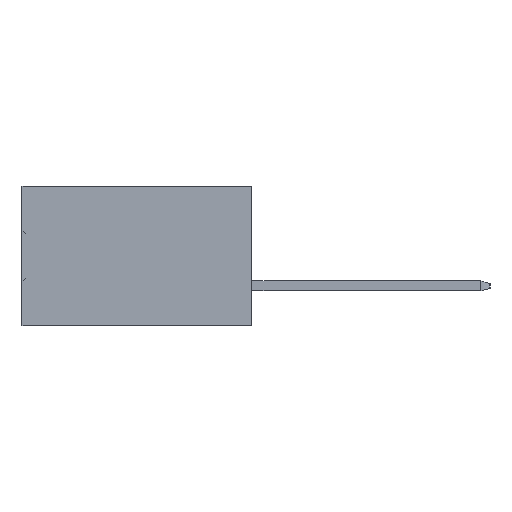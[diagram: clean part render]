
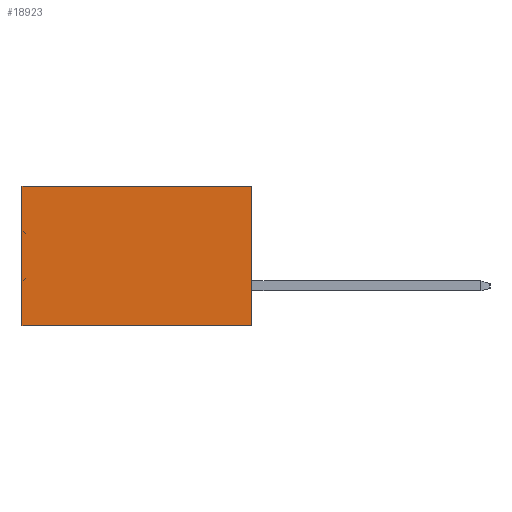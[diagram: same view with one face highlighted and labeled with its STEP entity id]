
A CAD part, left-side view. The second image highlights one B-rep face of the part: STEP entity #18923.
In plain terms, the highlighted planar face has unit normal (-1, 0, 0).
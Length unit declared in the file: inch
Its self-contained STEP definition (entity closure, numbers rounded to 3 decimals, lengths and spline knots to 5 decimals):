
#586 = EDGE_CURVE ( 'NONE', #1185, #763, #6253, .T. ) ;
#763 = VERTEX_POINT ( 'NONE', #26705 ) ;
#858 = VECTOR ( 'NONE', #3975, 39.37008 ) ;
#1001 = VERTEX_POINT ( 'NONE', #30029 ) ;
#1177 = VECTOR ( 'NONE', #13660, 39.37008 ) ;
#1185 = VERTEX_POINT ( 'NONE', #25461 ) ;
#1842 = VERTEX_POINT ( 'NONE', #13421 ) ;
#2240 = ORIENTED_EDGE ( 'NONE', *, *, #21522, .F. ) ;
#2920 = ORIENTED_EDGE ( 'NONE', *, *, #586, .T. ) ;
#3974 = AXIS2_PLACEMENT_3D ( 'NONE', #12595, #21846, #10302 ) ;
#3975 = DIRECTION ( 'NONE',  ( 0., 0., -1. ) ) ;
#4330 = EDGE_CURVE ( 'NONE', #1842, #763, #25556, .T. ) ;
#5971 = LINE ( 'NONE', #22097, #19605 ) ;
#6253 = LINE ( 'NONE', #15533, #858 ) ;
#10302 = DIRECTION ( 'NONE',  ( 0., 0., -1. ) ) ;
#11812 = LINE ( 'NONE', #27898, #1177 ) ;
#12595 = CARTESIAN_POINT ( 'NONE',  ( 0.3205, 0., -0.437 ) ) ;
#13421 = CARTESIAN_POINT ( 'NONE',  ( 0.3205, 0., -0.437 ) ) ;
#13660 = DIRECTION ( 'NONE',  ( 0., 0., -1. ) ) ;
#14871 = PLANE ( 'NONE',  #3974 ) ;
#15533 = CARTESIAN_POINT ( 'NONE',  ( 0.3205, 0.72, -0.437 ) ) ;
#18923 = ADVANCED_FACE ( 'NONE', ( #29416 ), #14871, .F. ) ;
#19605 = VECTOR ( 'NONE', #23816, 39.37008 ) ;
#20852 = CARTESIAN_POINT ( 'NONE',  ( 0.3205, 0., -0.437 ) ) ;
#21522 = EDGE_CURVE ( 'NONE', #1001, #1842, #11812, .T. ) ;
#21846 = DIRECTION ( 'NONE',  ( 1., 0., 0. ) ) ;
#22097 = CARTESIAN_POINT ( 'NONE',  ( 0.3205, 0., 0. ) ) ;
#23233 = EDGE_CURVE ( 'NONE', #1001, #1185, #5971, .T. ) ;
#23816 = DIRECTION ( 'NONE',  ( 0., 1., 0. ) ) ;
#25461 = CARTESIAN_POINT ( 'NONE',  ( 0.3205, 0.72, 0. ) ) ;
#25556 = LINE ( 'NONE', #20852, #27188 ) ;
#25699 = DIRECTION ( 'NONE',  ( 0., 1., 0. ) ) ;
#26705 = CARTESIAN_POINT ( 'NONE',  ( 0.3205, 0.72, -0.437 ) ) ;
#27188 = VECTOR ( 'NONE', #25699, 39.37008 ) ;
#27898 = CARTESIAN_POINT ( 'NONE',  ( 0.3205, 0., -0.437 ) ) ;
#28160 = ORIENTED_EDGE ( 'NONE', *, *, #4330, .F. ) ;
#28763 = ORIENTED_EDGE ( 'NONE', *, *, #23233, .T. ) ;
#29416 = FACE_OUTER_BOUND ( 'NONE', #29439, .T. ) ;
#29439 = EDGE_LOOP ( 'NONE', ( #2920, #28160, #2240, #28763 ) ) ;
#30029 = CARTESIAN_POINT ( 'NONE',  ( 0.3205, 0., 0. ) ) ;
